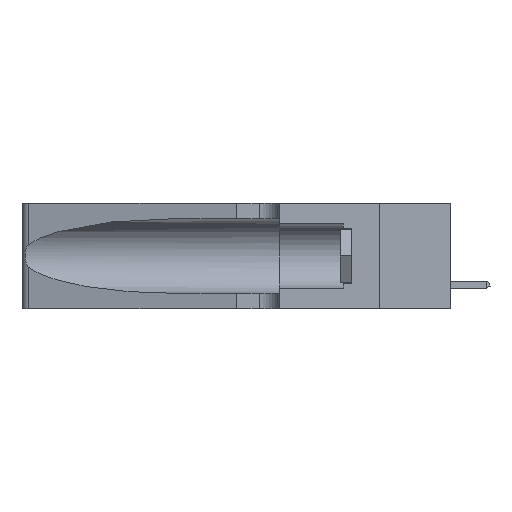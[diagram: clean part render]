
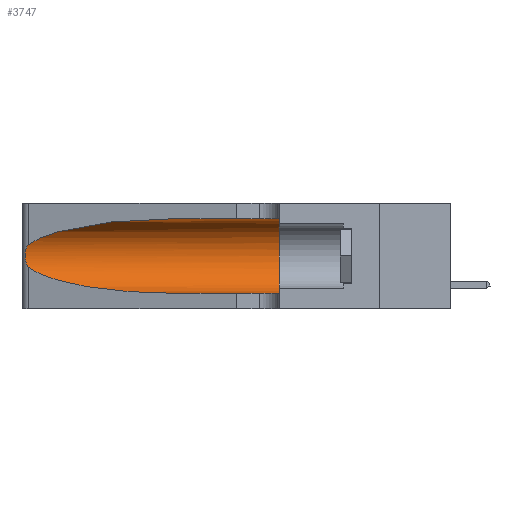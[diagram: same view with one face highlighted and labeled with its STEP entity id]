
A CAD part, left-side view. The second image highlights one B-rep face of the part: STEP entity #3747.
In plain terms, the highlighted cylindrical face has radius 3.308 mm (diameter 6.617 mm), a partial arc.
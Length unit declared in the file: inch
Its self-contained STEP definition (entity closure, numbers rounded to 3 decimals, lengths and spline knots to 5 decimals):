
#1311 = CARTESIAN_POINT ( 'NONE',  ( 0.25639, 1.23186, 0.15144 ) ) ;
#1461 = CARTESIAN_POINT ( 'NONE',  ( 0.25789, 1.23486, 0.15765 ) ) ;
#2026 = VERTEX_POINT ( 'NONE', #23356 ) ;
#3577 = ORIENTED_EDGE ( 'NONE', *, *, #21941, .T. ) ;
#3615 = CIRCLE ( 'NONE', #16775, 0.13025 ) ;
#3747 = ADVANCED_FACE ( 'NONE', ( #16338 ), #29414, .F. ) ;
#3789 = DIRECTION ( 'NONE',  ( 0., -1., 0. ) ) ;
#5578 = ORIENTED_EDGE ( 'NONE', *, *, #29621, .T. ) ;
#5934 = DIRECTION ( 'NONE',  ( 0., -1., 0. ) ) ;
#7193 = CARTESIAN_POINT ( 'NONE',  ( 0.25787, 1.23484, 0.2124 ) ) ;
#7319 = CARTESIAN_POINT ( 'NONE',  ( 0.25555, 1.22993, 0.14849 ) ) ;
#7959 = CARTESIAN_POINT ( 'NONE',  ( 0.25487, 1.22718, 0.14631 ) ) ;
#8027 = CARTESIAN_POINT ( 'NONE',  ( 0.1305, 0.72297, 0.31525 ) ) ;
#8074 = VERTEX_POINT ( 'NONE', #35486 ) ;
#8132 = CARTESIAN_POINT ( 'NONE',  ( 0.18966, 0.96281, 0.31525 ) ) ;
#8174 = VERTEX_POINT ( 'NONE', #38711 ) ;
#9806 = VECTOR ( 'NONE', #37651, 39.37008 ) ;
#11211 = CARTESIAN_POINT ( 'NONE',  ( 0.1305, 0.35, 0.05475 ) ) ;
#11914 = VERTEX_POINT ( 'NONE', #11211 ) ;
#12709 = CARTESIAN_POINT ( 'NONE',  ( 0.1305, 0.35, 0.185 ) ) ;
#13428 = CARTESIAN_POINT ( 'NONE',  ( 0.26075, 1.23896, 0.178 ) ) ;
#13520 =( BOUNDED_CURVE ( )  B_SPLINE_CURVE ( 3, ( #32239, #8132, #26130, #19827 ),
 .UNSPECIFIED., .F., .F. ) 
 B_SPLINE_CURVE_WITH_KNOTS ( ( 4, 4 ),
 ( 1.5708, 2.84003 ),
 .UNSPECIFIED. ) 
 CURVE ( )  GEOMETRIC_REPRESENTATION_ITEM ( )  RATIONAL_B_SPLINE_CURVE ( ( 1., 0.87, 0.87, 1. ) ) 
 REPRESENTATION_ITEM ( '' )  );
#15225 = AXIS2_PLACEMENT_3D ( 'NONE', #26909, #5934, #18152 ) ;
#15734 = DIRECTION ( 'NONE',  ( 0., 0., 1. ) ) ;
#16320 = CARTESIAN_POINT ( 'NONE',  ( 0.26075, 1.23896, 0.19203 ) ) ;
#16338 = FACE_OUTER_BOUND ( 'NONE', #23438, .T. ) ;
#16775 = AXIS2_PLACEMENT_3D ( 'NONE', #12709, #33648, #15734 ) ;
#18152 = DIRECTION ( 'NONE',  ( 0., 0., -1. ) ) ;
#18977 = EDGE_CURVE ( 'NONE', #35875, #2026, #26646, .T. ) ;
#19028 = CARTESIAN_POINT ( 'NONE',  ( 0.25555, 1.22994, 0.2215 ) ) ;
#19135 = CARTESIAN_POINT ( 'NONE',  ( 0.1305, 1.61858, 0.31525 ) ) ;
#19202 = EDGE_CURVE ( 'NONE', #23431, #8074, #23337, .T. ) ;
#19827 = CARTESIAN_POINT ( 'NONE',  ( 0.25487, 1.22718, 0.22369 ) ) ;
#19964 = EDGE_CURVE ( 'NONE', #35875, #23431, #13520, .T. ) ;
#20182 = CARTESIAN_POINT ( 'NONE',  ( 0.18966, 0.96281, 0.05475 ) ) ;
#21032 = EDGE_CURVE ( 'NONE', #2026, #11914, #3615, .T. ) ;
#21941 = EDGE_CURVE ( 'NONE', #8074, #8174, #22825, .T. ) ;
#22825 =( BOUNDED_CURVE ( )  B_SPLINE_CURVE ( 3, ( #7959, #28785, #20182, #29185 ),
 .UNSPECIFIED., .F., .F. ) 
 B_SPLINE_CURVE_WITH_KNOTS ( ( 4, 4 ),
 ( 3.44316, 4.71239 ),
 .UNSPECIFIED. ) 
 CURVE ( )  GEOMETRIC_REPRESENTATION_ITEM ( )  RATIONAL_B_SPLINE_CURVE ( ( 1., 0.87, 0.87, 1. ) ) 
 REPRESENTATION_ITEM ( '' )  );
#23337 = B_SPLINE_CURVE_WITH_KNOTS ( 'NONE', 3,
 ( #28435, #19028, #28187, #7193, #25158, #28046, #16320, #13428, #37128, #34110, #1461, #1311, #7319, #37266 ),
 .UNSPECIFIED., .F., .F.,
 ( 4, 2, 2, 2, 2, 2, 4 ),
 ( 0., 0.00027, 0.00053, 0.00107, 0.0016, 0.00187, 0.00214 ),
 .UNSPECIFIED. ) ;
#23356 = CARTESIAN_POINT ( 'NONE',  ( 0.1305, 0.35, 0.31525 ) ) ;
#23431 = VERTEX_POINT ( 'NONE', #28724 ) ;
#23438 = EDGE_LOOP ( 'NONE', ( #36848, #23867, #3577, #5578, #26939, #23850 ) ) ;
#23850 = ORIENTED_EDGE ( 'NONE', *, *, #18977, .F. ) ;
#23867 = ORIENTED_EDGE ( 'NONE', *, *, #19202, .T. ) ;
#23993 = CARTESIAN_POINT ( 'NONE',  ( 0.1305, 1.61858, 0.05475 ) ) ;
#25158 = CARTESIAN_POINT ( 'NONE',  ( 0.25854, 1.2359, 0.20912 ) ) ;
#26130 = CARTESIAN_POINT ( 'NONE',  ( 0.2373, 1.15595, 0.28018 ) ) ;
#26646 = LINE ( 'NONE', #19135, #9806 ) ;
#26909 = CARTESIAN_POINT ( 'NONE',  ( 0.1305, 1.61858, 0.185 ) ) ;
#26939 = ORIENTED_EDGE ( 'NONE', *, *, #21032, .F. ) ;
#27805 = VECTOR ( 'NONE', #3789, 39.37008 ) ;
#28046 = CARTESIAN_POINT ( 'NONE',  ( 0.26018, 1.23835, 0.19895 ) ) ;
#28187 = CARTESIAN_POINT ( 'NONE',  ( 0.25639, 1.23184, 0.21858 ) ) ;
#28435 = CARTESIAN_POINT ( 'NONE',  ( 0.25487, 1.22718, 0.22369 ) ) ;
#28724 = CARTESIAN_POINT ( 'NONE',  ( 0.25487, 1.22718, 0.22369 ) ) ;
#28785 = CARTESIAN_POINT ( 'NONE',  ( 0.2373, 1.15595, 0.08982 ) ) ;
#29185 = CARTESIAN_POINT ( 'NONE',  ( 0.1305, 0.72297, 0.05475 ) ) ;
#29414 = CYLINDRICAL_SURFACE ( 'NONE', #15225, 0.13025 ) ;
#29621 = EDGE_CURVE ( 'NONE', #8174, #11914, #33923, .T. ) ;
#32239 = CARTESIAN_POINT ( 'NONE',  ( 0.1305, 0.72297, 0.31525 ) ) ;
#33648 = DIRECTION ( 'NONE',  ( 0., 1., 0. ) ) ;
#33923 = LINE ( 'NONE', #23993, #27805 ) ;
#34110 = CARTESIAN_POINT ( 'NONE',  ( 0.25856, 1.23593, 0.16098 ) ) ;
#35486 = CARTESIAN_POINT ( 'NONE',  ( 0.25487, 1.22718, 0.14631 ) ) ;
#35875 = VERTEX_POINT ( 'NONE', #8027 ) ;
#36848 = ORIENTED_EDGE ( 'NONE', *, *, #19964, .T. ) ;
#37128 = CARTESIAN_POINT ( 'NONE',  ( 0.26017, 1.23833, 0.17102 ) ) ;
#37266 = CARTESIAN_POINT ( 'NONE',  ( 0.25487, 1.22718, 0.14631 ) ) ;
#37651 = DIRECTION ( 'NONE',  ( 0., -1., 0. ) ) ;
#38711 = CARTESIAN_POINT ( 'NONE',  ( 0.1305, 0.72297, 0.05475 ) ) ;
